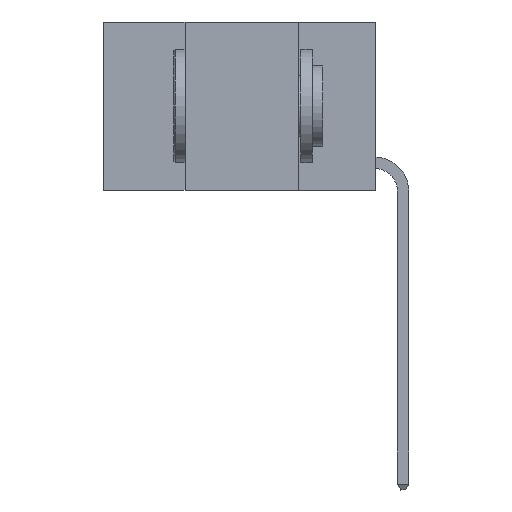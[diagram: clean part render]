
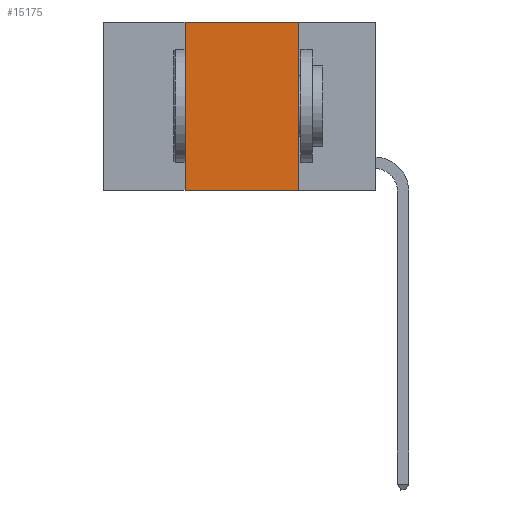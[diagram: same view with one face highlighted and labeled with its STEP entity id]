
A CAD part, left-side view. The second image highlights one B-rep face of the part: STEP entity #15175.
In plain terms, the highlighted planar face has unit normal (-1, 0, 0).
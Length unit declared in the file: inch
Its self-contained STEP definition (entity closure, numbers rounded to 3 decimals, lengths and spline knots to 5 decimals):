
#85 = LINE ( 'NONE', #5064, #9072 ) ;
#637 = VECTOR ( 'NONE', #2749, 39.37008 ) ;
#1602 = VECTOR ( 'NONE', #6276, 39.37008 ) ;
#2681 = ORIENTED_EDGE ( 'NONE', *, *, #16099, .T. ) ;
#2749 = DIRECTION ( 'NONE',  ( 0., 0., 1. ) ) ;
#3059 = PLANE ( 'NONE',  #4810 ) ;
#3139 = DIRECTION ( 'NONE',  ( 0., 0., -1. ) ) ;
#3401 = VECTOR ( 'NONE', #4210, 39.37008 ) ;
#3926 = CARTESIAN_POINT ( 'NONE',  ( 0., 0.6, -0.37 ) ) ;
#4104 = ORIENTED_EDGE ( 'NONE', *, *, #12375, .F. ) ;
#4210 = DIRECTION ( 'NONE',  ( 0., -1., 0. ) ) ;
#4810 = AXIS2_PLACEMENT_3D ( 'NONE', #13323, #12206, #3139 ) ;
#5064 = CARTESIAN_POINT ( 'NONE',  ( 0., 0.17, 0. ) ) ;
#5195 = CARTESIAN_POINT ( 'NONE',  ( 0., 0.42, 0. ) ) ;
#5594 = ORIENTED_EDGE ( 'NONE', *, *, #8786, .F. ) ;
#6113 = VERTEX_POINT ( 'NONE', #8631 ) ;
#6276 = DIRECTION ( 'NONE',  ( 0., -1., 0. ) ) ;
#6280 = CARTESIAN_POINT ( 'NONE',  ( 0., 0.42, -0.37 ) ) ;
#6465 = LINE ( 'NONE', #9217, #3401 ) ;
#6564 = VERTEX_POINT ( 'NONE', #11308 ) ;
#7070 = FACE_OUTER_BOUND ( 'NONE', #8771, .T. ) ;
#7292 = CARTESIAN_POINT ( 'NONE',  ( 0., 0.17, -0.37 ) ) ;
#8631 = CARTESIAN_POINT ( 'NONE',  ( 0., 0.42, 0. ) ) ;
#8771 = EDGE_LOOP ( 'NONE', ( #11942, #4104, #5594, #2681 ) ) ;
#8786 = EDGE_CURVE ( 'NONE', #14135, #6113, #16576, .T. ) ;
#9072 = VECTOR ( 'NONE', #15253, 39.37008 ) ;
#9217 = CARTESIAN_POINT ( 'NONE',  ( 0., 0.6, 0. ) ) ;
#11308 = CARTESIAN_POINT ( 'NONE',  ( 0., 0.17, 0. ) ) ;
#11942 = ORIENTED_EDGE ( 'NONE', *, *, #15486, .F. ) ;
#12206 = DIRECTION ( 'NONE',  ( 1., 0., 0. ) ) ;
#12375 = EDGE_CURVE ( 'NONE', #6113, #6564, #6465, .T. ) ;
#13323 = CARTESIAN_POINT ( 'NONE',  ( 0., 0.6, 0. ) ) ;
#14000 = VERTEX_POINT ( 'NONE', #7292 ) ;
#14135 = VERTEX_POINT ( 'NONE', #6280 ) ;
#15175 = ADVANCED_FACE ( 'NONE', ( #7070 ), #3059, .F. ) ;
#15253 = DIRECTION ( 'NONE',  ( 0., 0., -1. ) ) ;
#15464 = LINE ( 'NONE', #3926, #1602 ) ;
#15486 = EDGE_CURVE ( 'NONE', #6564, #14000, #85, .T. ) ;
#16099 = EDGE_CURVE ( 'NONE', #14135, #14000, #15464, .T. ) ;
#16576 = LINE ( 'NONE', #5195, #637 ) ;
